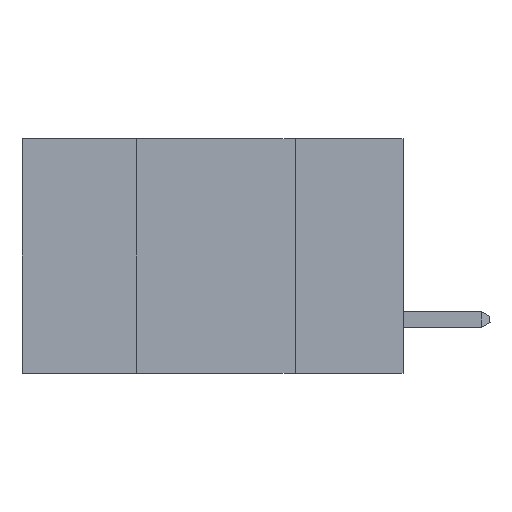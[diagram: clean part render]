
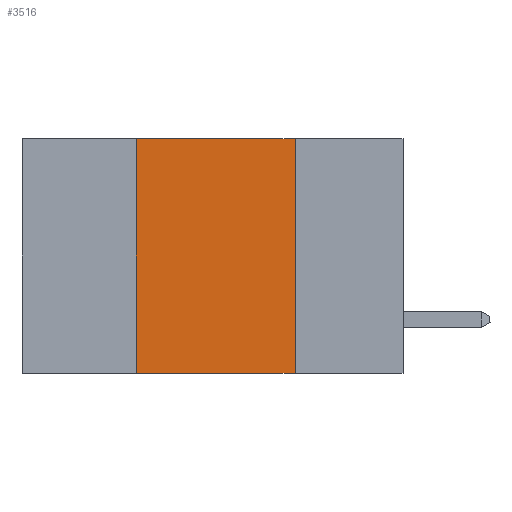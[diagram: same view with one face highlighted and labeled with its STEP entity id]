
A CAD part, left-side view. The second image highlights one B-rep face of the part: STEP entity #3516.
In plain terms, the highlighted planar face has unit normal (-1, 0, 0).
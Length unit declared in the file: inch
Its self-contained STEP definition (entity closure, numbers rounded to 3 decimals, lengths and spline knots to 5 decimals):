
#172 = ORIENTED_EDGE ( 'NONE', *, *, #10469, .F. ) ;
#223 = VECTOR ( 'NONE', #7072, 39.37008 ) ;
#340 = PLANE ( 'NONE',  #2635 ) ;
#534 = LINE ( 'NONE', #2580, #5302 ) ;
#880 = CARTESIAN_POINT ( 'NONE',  ( 0., 0.6, 0. ) ) ;
#1242 = CARTESIAN_POINT ( 'NONE',  ( 0., 0.42, -0.37 ) ) ;
#2050 = VERTEX_POINT ( 'NONE', #4470 ) ;
#2580 = CARTESIAN_POINT ( 'NONE',  ( 0., 0.17, 0. ) ) ;
#2635 = AXIS2_PLACEMENT_3D ( 'NONE', #5947, #8664, #9595 ) ;
#2694 = LINE ( 'NONE', #880, #9792 ) ;
#2801 = EDGE_CURVE ( 'NONE', #10602, #4122, #10559, .T. ) ;
#2877 = EDGE_LOOP ( 'NONE', ( #172, #10787, #8193, #6115 ) ) ;
#3516 = ADVANCED_FACE ( 'NONE', ( #6782 ), #340, .F. ) ;
#3540 = DIRECTION ( 'NONE',  ( 0., 0., -1. ) ) ;
#4122 = VERTEX_POINT ( 'NONE', #10010 ) ;
#4470 = CARTESIAN_POINT ( 'NONE',  ( 0., 0.17, -0.37 ) ) ;
#5302 = VECTOR ( 'NONE', #3540, 39.37008 ) ;
#5947 = CARTESIAN_POINT ( 'NONE',  ( 0., 0.6, 0. ) ) ;
#6115 = ORIENTED_EDGE ( 'NONE', *, *, #6220, .T. ) ;
#6220 = EDGE_CURVE ( 'NONE', #10602, #2050, #7154, .T. ) ;
#6782 = FACE_OUTER_BOUND ( 'NONE', #2877, .T. ) ;
#7072 = DIRECTION ( 'NONE',  ( 0., -1., 0. ) ) ;
#7154 = LINE ( 'NONE', #8092, #223 ) ;
#7347 = DIRECTION ( 'NONE',  ( 0., -1., 0. ) ) ;
#7804 = DIRECTION ( 'NONE',  ( 0., 0., 1. ) ) ;
#8092 = CARTESIAN_POINT ( 'NONE',  ( 0., 0.6, -0.37 ) ) ;
#8094 = VECTOR ( 'NONE', #7804, 39.37008 ) ;
#8193 = ORIENTED_EDGE ( 'NONE', *, *, #2801, .F. ) ;
#8664 = DIRECTION ( 'NONE',  ( 1., 0., 0. ) ) ;
#9595 = DIRECTION ( 'NONE',  ( 0., 0., -1. ) ) ;
#9623 = CARTESIAN_POINT ( 'NONE',  ( 0., 0.17, 0. ) ) ;
#9788 = EDGE_CURVE ( 'NONE', #4122, #10257, #2694, .T. ) ;
#9792 = VECTOR ( 'NONE', #7347, 39.37008 ) ;
#10010 = CARTESIAN_POINT ( 'NONE',  ( 0., 0.42, 0. ) ) ;
#10257 = VERTEX_POINT ( 'NONE', #9623 ) ;
#10469 = EDGE_CURVE ( 'NONE', #10257, #2050, #534, .T. ) ;
#10559 = LINE ( 'NONE', #11504, #8094 ) ;
#10602 = VERTEX_POINT ( 'NONE', #1242 ) ;
#10787 = ORIENTED_EDGE ( 'NONE', *, *, #9788, .F. ) ;
#11504 = CARTESIAN_POINT ( 'NONE',  ( 0., 0.42, 0. ) ) ;
